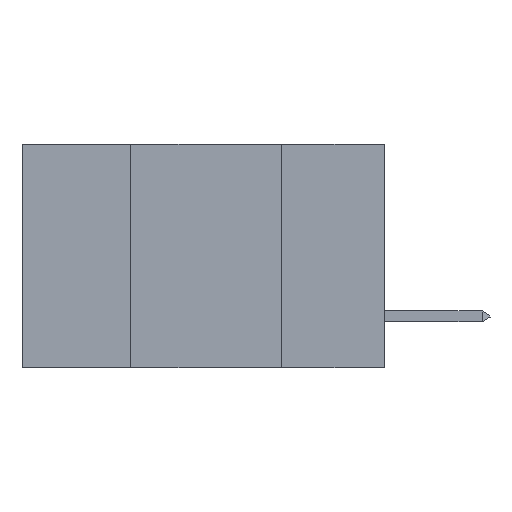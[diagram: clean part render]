
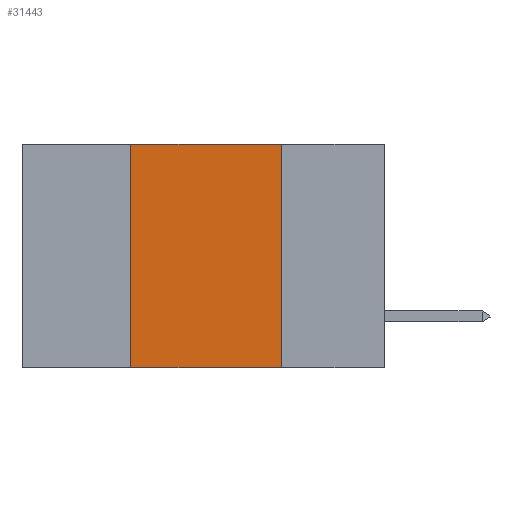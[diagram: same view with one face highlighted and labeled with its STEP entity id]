
A CAD part, left-side view. The second image highlights one B-rep face of the part: STEP entity #31443.
In plain terms, the highlighted planar face has unit normal (-1, 0, 0).
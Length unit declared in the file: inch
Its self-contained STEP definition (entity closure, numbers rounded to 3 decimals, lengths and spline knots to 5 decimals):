
#578 = CARTESIAN_POINT ( 'NONE',  ( 0., 0.17, 0. ) ) ;
#1881 = EDGE_LOOP ( 'NONE', ( #28061, #30899, #12284, #14650 ) ) ;
#2234 = VECTOR ( 'NONE', #13840, 39.37008 ) ;
#3013 = CARTESIAN_POINT ( 'NONE',  ( 0., 0.42, 0. ) ) ;
#3150 = VECTOR ( 'NONE', #18715, 39.37008 ) ;
#3182 = LINE ( 'NONE', #24952, #14367 ) ;
#3657 = EDGE_CURVE ( 'NONE', #33963, #21886, #14735, .T. ) ;
#5370 = CARTESIAN_POINT ( 'NONE',  ( 0., 0.42, -0.37 ) ) ;
#5541 = LINE ( 'NONE', #19405, #2234 ) ;
#5677 = PLANE ( 'NONE',  #24969 ) ;
#8130 = DIRECTION ( 'NONE',  ( 0., -1., 0. ) ) ;
#8265 = DIRECTION ( 'NONE',  ( 0., 0., -1. ) ) ;
#9114 = FACE_OUTER_BOUND ( 'NONE', #1881, .T. ) ;
#12284 = ORIENTED_EDGE ( 'NONE', *, *, #3657, .F. ) ;
#13581 = LINE ( 'NONE', #17715, #31810 ) ;
#13840 = DIRECTION ( 'NONE',  ( 0., 0., -1. ) ) ;
#14126 = EDGE_CURVE ( 'NONE', #21886, #22441, #13581, .T. ) ;
#14367 = VECTOR ( 'NONE', #25066, 39.37008 ) ;
#14650 = ORIENTED_EDGE ( 'NONE', *, *, #33572, .T. ) ;
#14735 = LINE ( 'NONE', #28901, #3150 ) ;
#17715 = CARTESIAN_POINT ( 'NONE',  ( 0., 0.6, 0. ) ) ;
#18715 = DIRECTION ( 'NONE',  ( 0., 0., 1. ) ) ;
#19405 = CARTESIAN_POINT ( 'NONE',  ( 0., 0.17, 0. ) ) ;
#21308 = CARTESIAN_POINT ( 'NONE',  ( 0., 0.6, 0. ) ) ;
#21886 = VERTEX_POINT ( 'NONE', #3013 ) ;
#22441 = VERTEX_POINT ( 'NONE', #578 ) ;
#23114 = EDGE_CURVE ( 'NONE', #22441, #26266, #5541, .T. ) ;
#24086 = DIRECTION ( 'NONE',  ( 1., 0., 0. ) ) ;
#24325 = CARTESIAN_POINT ( 'NONE',  ( 0., 0.17, -0.37 ) ) ;
#24952 = CARTESIAN_POINT ( 'NONE',  ( 0., 0.6, -0.37 ) ) ;
#24969 = AXIS2_PLACEMENT_3D ( 'NONE', #21308, #24086, #8265 ) ;
#25066 = DIRECTION ( 'NONE',  ( 0., -1., 0. ) ) ;
#26266 = VERTEX_POINT ( 'NONE', #24325 ) ;
#28061 = ORIENTED_EDGE ( 'NONE', *, *, #23114, .F. ) ;
#28901 = CARTESIAN_POINT ( 'NONE',  ( 0., 0.42, 0. ) ) ;
#30899 = ORIENTED_EDGE ( 'NONE', *, *, #14126, .F. ) ;
#31443 = ADVANCED_FACE ( 'NONE', ( #9114 ), #5677, .F. ) ;
#31810 = VECTOR ( 'NONE', #8130, 39.37008 ) ;
#33572 = EDGE_CURVE ( 'NONE', #33963, #26266, #3182, .T. ) ;
#33963 = VERTEX_POINT ( 'NONE', #5370 ) ;
